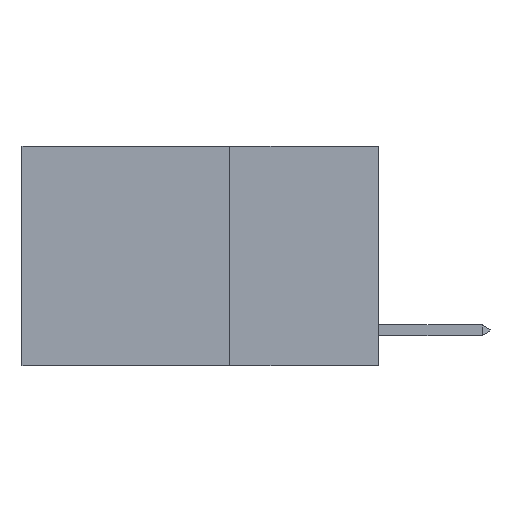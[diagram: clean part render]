
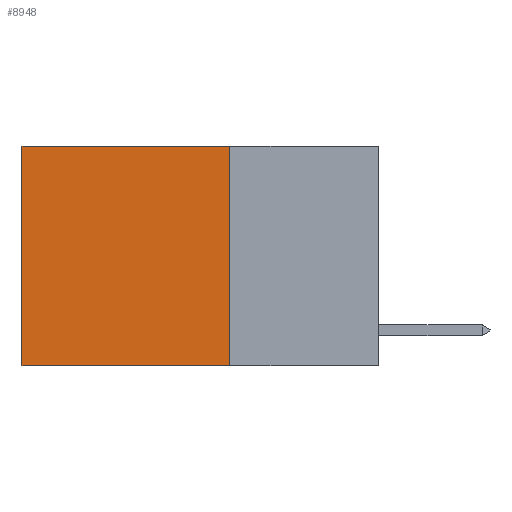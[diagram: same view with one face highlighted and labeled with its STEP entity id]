
A CAD part, left-side view. The second image highlights one B-rep face of the part: STEP entity #8948.
In plain terms, the highlighted planar face has unit normal (-1, 0, 0).
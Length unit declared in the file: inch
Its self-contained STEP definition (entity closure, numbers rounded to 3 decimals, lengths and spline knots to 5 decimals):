
#219 = EDGE_LOOP ( 'NONE', ( #5984, #4910, #1127, #6124 ) ) ;
#563 = CARTESIAN_POINT ( 'NONE',  ( 0.2625, 0.6, -0.37 ) ) ;
#892 = EDGE_CURVE ( 'NONE', #4887, #8248, #1909, .T. ) ;
#1057 = PLANE ( 'NONE',  #6705 ) ;
#1127 = ORIENTED_EDGE ( 'NONE', *, *, #8334, .F. ) ;
#1891 = CARTESIAN_POINT ( 'NONE',  ( 0.2625, 0.25, 0. ) ) ;
#1909 = LINE ( 'NONE', #3391, #7932 ) ;
#2113 = EDGE_CURVE ( 'NONE', #6251, #8248, #9394, .T. ) ;
#2115 = VECTOR ( 'NONE', #2488, 39.37008 ) ;
#2171 = VECTOR ( 'NONE', #9082, 39.37008 ) ;
#2488 = DIRECTION ( 'NONE',  ( 0., 1., 0. ) ) ;
#2986 = LINE ( 'NONE', #6830, #4312 ) ;
#3391 = CARTESIAN_POINT ( 'NONE',  ( 0.2625, 0.6, 0. ) ) ;
#3549 = DIRECTION ( 'NONE',  ( 0., 1., 0. ) ) ;
#3719 = EDGE_CURVE ( 'NONE', #6572, #4887, #2986, .T. ) ;
#3796 = CARTESIAN_POINT ( 'NONE',  ( 0.2625, 0.25, -0.37 ) ) ;
#4312 = VECTOR ( 'NONE', #3549, 39.37008 ) ;
#4427 = DIRECTION ( 'NONE',  ( 0., 0., -1. ) ) ;
#4887 = VERTEX_POINT ( 'NONE', #6632 ) ;
#4910 = ORIENTED_EDGE ( 'NONE', *, *, #2113, .F. ) ;
#5670 = FACE_OUTER_BOUND ( 'NONE', #219, .T. ) ;
#5739 = CARTESIAN_POINT ( 'NONE',  ( 0.2625, 0.25, 0. ) ) ;
#5984 = ORIENTED_EDGE ( 'NONE', *, *, #892, .T. ) ;
#6124 = ORIENTED_EDGE ( 'NONE', *, *, #3719, .T. ) ;
#6251 = VERTEX_POINT ( 'NONE', #3796 ) ;
#6572 = VERTEX_POINT ( 'NONE', #7835 ) ;
#6632 = CARTESIAN_POINT ( 'NONE',  ( 0.2625, 0.6, 0. ) ) ;
#6705 = AXIS2_PLACEMENT_3D ( 'NONE', #1891, #7733, #4427 ) ;
#6781 = DIRECTION ( 'NONE',  ( 0., 0., -1. ) ) ;
#6830 = CARTESIAN_POINT ( 'NONE',  ( 0.2625, 0.25, 0. ) ) ;
#7008 = LINE ( 'NONE', #5739, #2171 ) ;
#7510 = CARTESIAN_POINT ( 'NONE',  ( 0.2625, 0.25, -0.37 ) ) ;
#7733 = DIRECTION ( 'NONE',  ( 1., 0., 0. ) ) ;
#7835 = CARTESIAN_POINT ( 'NONE',  ( 0.2625, 0.25, 0. ) ) ;
#7932 = VECTOR ( 'NONE', #6781, 39.37008 ) ;
#8248 = VERTEX_POINT ( 'NONE', #563 ) ;
#8334 = EDGE_CURVE ( 'NONE', #6572, #6251, #7008, .T. ) ;
#8948 = ADVANCED_FACE ( 'NONE', ( #5670 ), #1057, .F. ) ;
#9082 = DIRECTION ( 'NONE',  ( 0., 0., -1. ) ) ;
#9394 = LINE ( 'NONE', #7510, #2115 ) ;
